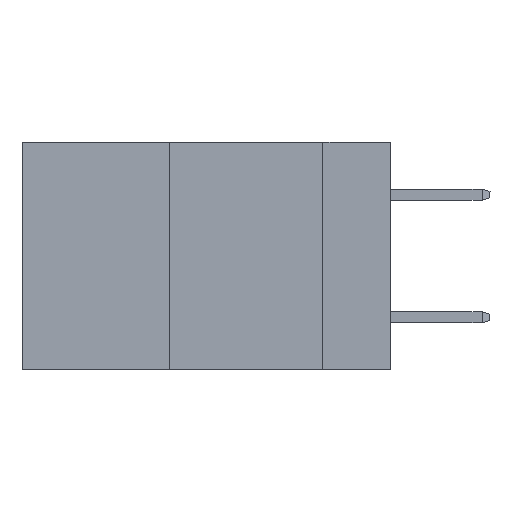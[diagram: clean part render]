
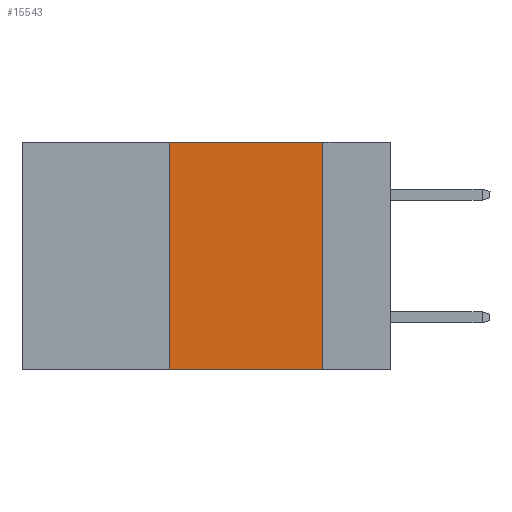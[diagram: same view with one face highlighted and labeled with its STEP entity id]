
A CAD part, left-side view. The second image highlights one B-rep face of the part: STEP entity #15543.
In plain terms, the highlighted planar face has unit normal (-1, 0, 0).
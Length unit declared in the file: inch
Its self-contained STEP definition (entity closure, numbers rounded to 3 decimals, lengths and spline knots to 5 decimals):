
#1353 = EDGE_CURVE ( 'NONE', #6218, #1981, #10771, .T. ) ;
#1981 = VERTEX_POINT ( 'NONE', #2299 ) ;
#2117 = ORIENTED_EDGE ( 'NONE', *, *, #8345, .F. ) ;
#2299 = CARTESIAN_POINT ( 'NONE',  ( 0., 0.11, -0.37 ) ) ;
#2490 = FACE_OUTER_BOUND ( 'NONE', #3427, .T. ) ;
#3427 = EDGE_LOOP ( 'NONE', ( #11346, #12156, #2117, #15888 ) ) ;
#3495 = VERTEX_POINT ( 'NONE', #4213 ) ;
#3820 = VECTOR ( 'NONE', #13077, 39.37008 ) ;
#4213 = CARTESIAN_POINT ( 'NONE',  ( 0., 0.36, 0. ) ) ;
#4781 = DIRECTION ( 'NONE',  ( 0., 0., -1. ) ) ;
#4942 = CARTESIAN_POINT ( 'NONE',  ( 0., 0.6, 0. ) ) ;
#5867 = DIRECTION ( 'NONE',  ( 1., 0., 0. ) ) ;
#5916 = DIRECTION ( 'NONE',  ( 0., 0., 1. ) ) ;
#6092 = CARTESIAN_POINT ( 'NONE',  ( 0., 0.11, 0. ) ) ;
#6200 = CARTESIAN_POINT ( 'NONE',  ( 0., 0.11, 0. ) ) ;
#6218 = VERTEX_POINT ( 'NONE', #15654 ) ;
#6249 = DIRECTION ( 'NONE',  ( 0., -1., 0. ) ) ;
#6577 = VERTEX_POINT ( 'NONE', #6200 ) ;
#8216 = VECTOR ( 'NONE', #5916, 39.37008 ) ;
#8345 = EDGE_CURVE ( 'NONE', #6218, #3495, #8609, .T. ) ;
#8402 = VECTOR ( 'NONE', #6249, 39.37008 ) ;
#8529 = EDGE_CURVE ( 'NONE', #3495, #6577, #15595, .T. ) ;
#8609 = LINE ( 'NONE', #13599, #8216 ) ;
#9700 = CARTESIAN_POINT ( 'NONE',  ( 0., 0.6, 0. ) ) ;
#10771 = LINE ( 'NONE', #12439, #3820 ) ;
#11346 = ORIENTED_EDGE ( 'NONE', *, *, #12657, .F. ) ;
#12156 = ORIENTED_EDGE ( 'NONE', *, *, #8529, .F. ) ;
#12439 = CARTESIAN_POINT ( 'NONE',  ( 0., 0.6, -0.37 ) ) ;
#12657 = EDGE_CURVE ( 'NONE', #6577, #1981, #13976, .T. ) ;
#13077 = DIRECTION ( 'NONE',  ( 0., -1., 0. ) ) ;
#13552 = PLANE ( 'NONE',  #14295 ) ;
#13599 = CARTESIAN_POINT ( 'NONE',  ( 0., 0.36, 0. ) ) ;
#13976 = LINE ( 'NONE', #6092, #16509 ) ;
#14295 = AXIS2_PLACEMENT_3D ( 'NONE', #9700, #5867, #14832 ) ;
#14832 = DIRECTION ( 'NONE',  ( 0., 0., -1. ) ) ;
#15543 = ADVANCED_FACE ( 'NONE', ( #2490 ), #13552, .F. ) ;
#15595 = LINE ( 'NONE', #4942, #8402 ) ;
#15654 = CARTESIAN_POINT ( 'NONE',  ( 0., 0.36, -0.37 ) ) ;
#15888 = ORIENTED_EDGE ( 'NONE', *, *, #1353, .T. ) ;
#16509 = VECTOR ( 'NONE', #4781, 39.37008 ) ;
